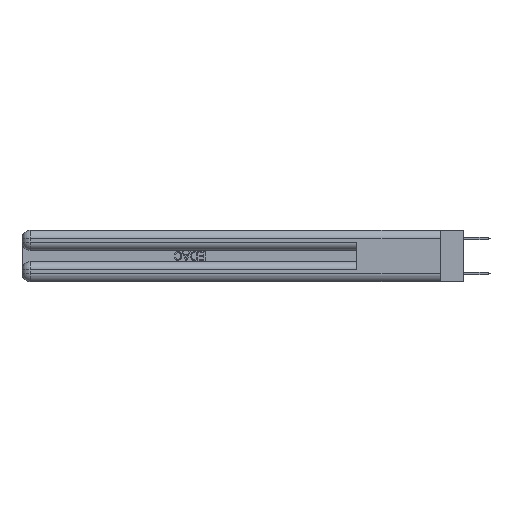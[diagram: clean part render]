
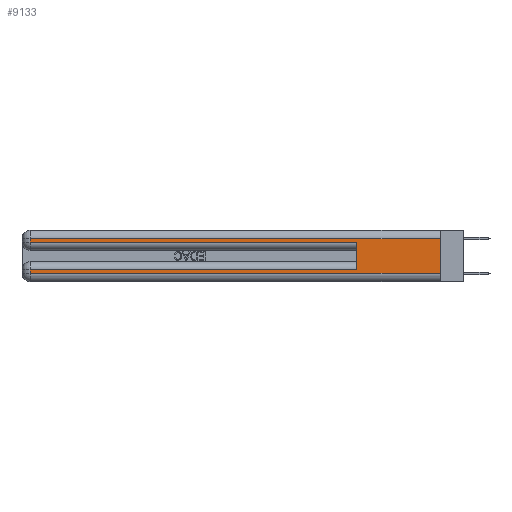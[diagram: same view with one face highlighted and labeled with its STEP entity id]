
A CAD part, left-side view. The second image highlights one B-rep face of the part: STEP entity #9133.
In plain terms, the highlighted planar face has unit normal (-1, 0, 0).
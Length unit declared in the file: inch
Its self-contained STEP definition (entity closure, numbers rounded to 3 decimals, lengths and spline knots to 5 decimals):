
#1427 = LINE ( 'NONE', #26849, #17187 ) ;
#1732 = DIRECTION ( 'NONE',  ( 0., 1., 0. ) ) ;
#2045 = EDGE_CURVE ( 'NONE', #8011, #26975, #27166, .T. ) ;
#2430 = CARTESIAN_POINT ( 'NONE',  ( 0., 2.94, 0.085 ) ) ;
#3193 = LINE ( 'NONE', #12935, #29019 ) ;
#3210 = DIRECTION ( 'NONE',  ( 0., 0., 1. ) ) ;
#3717 = ORIENTED_EDGE ( 'NONE', *, *, #21248, .T. ) ;
#4566 = VERTEX_POINT ( 'NONE', #24009 ) ;
#4947 = ORIENTED_EDGE ( 'NONE', *, *, #19868, .T. ) ;
#5209 = LINE ( 'NONE', #10022, #18975 ) ;
#6497 = ORIENTED_EDGE ( 'NONE', *, *, #15863, .T. ) ;
#8011 = VERTEX_POINT ( 'NONE', #18141 ) ;
#8300 = CARTESIAN_POINT ( 'NONE',  ( 0., 0.6, 0.285 ) ) ;
#9133 = ADVANCED_FACE ( 'NONE', ( #19338 ), #11803, .F. ) ;
#9510 = DIRECTION ( 'NONE',  ( 1., 0., 0. ) ) ;
#9875 = DIRECTION ( 'NONE',  ( 0., 0., -1. ) ) ;
#9910 = ORIENTED_EDGE ( 'NONE', *, *, #20463, .F. ) ;
#10022 = CARTESIAN_POINT ( 'NONE',  ( 0., 2.94, 0.37 ) ) ;
#10088 = DIRECTION ( 'NONE',  ( 0., 0., -1. ) ) ;
#10263 = VECTOR ( 'NONE', #17670, 39.37008 ) ;
#10273 = VERTEX_POINT ( 'NONE', #27903 ) ;
#11372 = DIRECTION ( 'NONE',  ( 0., 1., 0. ) ) ;
#11644 = DIRECTION ( 'NONE',  ( 0., 0., -1. ) ) ;
#11803 = PLANE ( 'NONE',  #17356 ) ;
#12935 = CARTESIAN_POINT ( 'NONE',  ( 0., 2.94, 0.37 ) ) ;
#13805 = LINE ( 'NONE', #22874, #27470 ) ;
#14251 = DIRECTION ( 'NONE',  ( 0., -1., 0. ) ) ;
#14382 = ORIENTED_EDGE ( 'NONE', *, *, #2045, .F. ) ;
#14545 = EDGE_LOOP ( 'NONE', ( #14382, #16591, #22628, #4947, #9910, #3717, #6497, #29204 ) ) ;
#14547 = VECTOR ( 'NONE', #11644, 39.37008 ) ;
#15127 = CARTESIAN_POINT ( 'NONE',  ( 0., 0., 0.06 ) ) ;
#15341 = CARTESIAN_POINT ( 'NONE',  ( 0., 2.94, 0.06 ) ) ;
#15863 = EDGE_CURVE ( 'NONE', #18734, #24697, #3193, .T. ) ;
#16591 = ORIENTED_EDGE ( 'NONE', *, *, #26881, .T. ) ;
#17141 = VERTEX_POINT ( 'NONE', #28612 ) ;
#17187 = VECTOR ( 'NONE', #1732, 39.37008 ) ;
#17262 = EDGE_CURVE ( 'NONE', #24697, #26975, #24727, .T. ) ;
#17356 = AXIS2_PLACEMENT_3D ( 'NONE', #21026, #9510, #18897 ) ;
#17531 = VECTOR ( 'NONE', #14251, 39.37008 ) ;
#17670 = DIRECTION ( 'NONE',  ( 0., -1., 0. ) ) ;
#18141 = CARTESIAN_POINT ( 'NONE',  ( 0., 0., 0.31 ) ) ;
#18734 = VERTEX_POINT ( 'NONE', #2430 ) ;
#18897 = DIRECTION ( 'NONE',  ( 0., 0., -1. ) ) ;
#18975 = VECTOR ( 'NONE', #9875, 39.37008 ) ;
#19338 = FACE_OUTER_BOUND ( 'NONE', #14545, .T. ) ;
#19472 = EDGE_CURVE ( 'NONE', #4566, #10273, #5209, .T. ) ;
#19868 = EDGE_CURVE ( 'NONE', #10273, #22164, #28216, .T. ) ;
#20426 = CARTESIAN_POINT ( 'NONE',  ( 0., 0., 0.37 ) ) ;
#20463 = EDGE_CURVE ( 'NONE', #17141, #22164, #24145, .T. ) ;
#20603 = CARTESIAN_POINT ( 'NONE',  ( 0., 0., 0.06 ) ) ;
#21026 = CARTESIAN_POINT ( 'NONE',  ( 0., 0., 0.37 ) ) ;
#21248 = EDGE_CURVE ( 'NONE', #17141, #18734, #1427, .T. ) ;
#22164 = VERTEX_POINT ( 'NONE', #8300 ) ;
#22628 = ORIENTED_EDGE ( 'NONE', *, *, #19472, .T. ) ;
#22874 = CARTESIAN_POINT ( 'NONE',  ( 0., 0., 0.31 ) ) ;
#23303 = CARTESIAN_POINT ( 'NONE',  ( 0., 0., 0.285 ) ) ;
#24009 = CARTESIAN_POINT ( 'NONE',  ( 0., 2.94, 0.31 ) ) ;
#24145 = LINE ( 'NONE', #26094, #29023 ) ;
#24697 = VERTEX_POINT ( 'NONE', #15341 ) ;
#24727 = LINE ( 'NONE', #15127, #10263 ) ;
#26094 = CARTESIAN_POINT ( 'NONE',  ( 0., 0.6, 0.145 ) ) ;
#26849 = CARTESIAN_POINT ( 'NONE',  ( 0., 0., 0.085 ) ) ;
#26881 = EDGE_CURVE ( 'NONE', #8011, #4566, #13805, .T. ) ;
#26975 = VERTEX_POINT ( 'NONE', #20603 ) ;
#27166 = LINE ( 'NONE', #20426, #14547 ) ;
#27470 = VECTOR ( 'NONE', #11372, 39.37008 ) ;
#27903 = CARTESIAN_POINT ( 'NONE',  ( 0., 2.94, 0.285 ) ) ;
#28216 = LINE ( 'NONE', #23303, #17531 ) ;
#28612 = CARTESIAN_POINT ( 'NONE',  ( 0., 0.6, 0.085 ) ) ;
#29019 = VECTOR ( 'NONE', #10088, 39.37008 ) ;
#29023 = VECTOR ( 'NONE', #3210, 39.37008 ) ;
#29204 = ORIENTED_EDGE ( 'NONE', *, *, #17262, .T. ) ;
